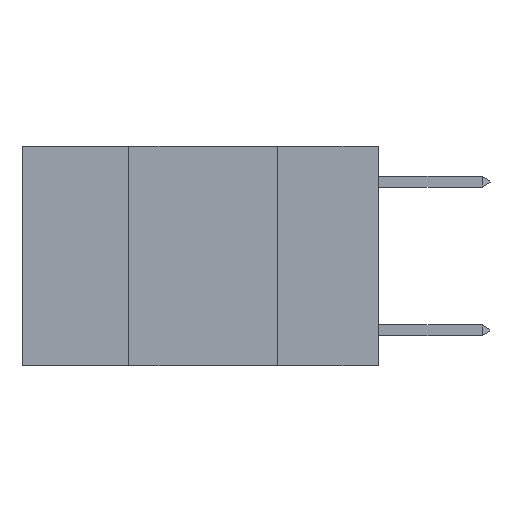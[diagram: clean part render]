
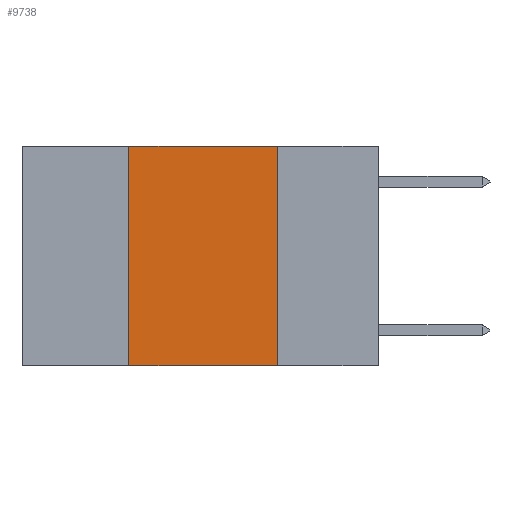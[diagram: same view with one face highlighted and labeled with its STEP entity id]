
A CAD part, left-side view. The second image highlights one B-rep face of the part: STEP entity #9738.
In plain terms, the highlighted planar face has unit normal (-1, 0, 0).
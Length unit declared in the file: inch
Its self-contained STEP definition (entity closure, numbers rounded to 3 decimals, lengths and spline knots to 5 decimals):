
#748 = VERTEX_POINT ( 'NONE', #5914 ) ;
#987 = CARTESIAN_POINT ( 'NONE',  ( 0., 0.17, -0.37 ) ) ;
#1013 = PLANE ( 'NONE',  #9119 ) ;
#1618 = DIRECTION ( 'NONE',  ( 0., 0., 1. ) ) ;
#1812 = DIRECTION ( 'NONE',  ( 1., 0., 0. ) ) ;
#1845 = CARTESIAN_POINT ( 'NONE',  ( 0., 0.6, -0.37 ) ) ;
#1848 = EDGE_CURVE ( 'NONE', #4637, #2134, #8633, .T. ) ;
#2129 = ORIENTED_EDGE ( 'NONE', *, *, #1848, .F. ) ;
#2134 = VERTEX_POINT ( 'NONE', #987 ) ;
#2303 = EDGE_CURVE ( 'NONE', #7152, #748, #2672, .T. ) ;
#2428 = VECTOR ( 'NONE', #5171, 39.37008 ) ;
#2672 = LINE ( 'NONE', #6162, #8623 ) ;
#2759 = ORIENTED_EDGE ( 'NONE', *, *, #5138, .F. ) ;
#2793 = EDGE_LOOP ( 'NONE', ( #2129, #2759, #3598, #3946 ) ) ;
#3598 = ORIENTED_EDGE ( 'NONE', *, *, #2303, .F. ) ;
#3946 = ORIENTED_EDGE ( 'NONE', *, *, #9270, .T. ) ;
#4184 = DIRECTION ( 'NONE',  ( 0., -1., 0. ) ) ;
#4637 = VERTEX_POINT ( 'NONE', #9753 ) ;
#5138 = EDGE_CURVE ( 'NONE', #748, #4637, #8863, .T. ) ;
#5171 = DIRECTION ( 'NONE',  ( 0., 0., -1. ) ) ;
#5399 = VECTOR ( 'NONE', #6515, 39.37008 ) ;
#5540 = CARTESIAN_POINT ( 'NONE',  ( 0., 0.42, -0.37 ) ) ;
#5815 = CARTESIAN_POINT ( 'NONE',  ( 0., 0.17, 0. ) ) ;
#5914 = CARTESIAN_POINT ( 'NONE',  ( 0., 0.42, 0. ) ) ;
#6162 = CARTESIAN_POINT ( 'NONE',  ( 0., 0.42, 0. ) ) ;
#6515 = DIRECTION ( 'NONE',  ( 0., -1., 0. ) ) ;
#6570 = VECTOR ( 'NONE', #4184, 39.37008 ) ;
#7152 = VERTEX_POINT ( 'NONE', #5540 ) ;
#7278 = DIRECTION ( 'NONE',  ( 0., 0., -1. ) ) ;
#8080 = CARTESIAN_POINT ( 'NONE',  ( 0., 0.6, 0. ) ) ;
#8623 = VECTOR ( 'NONE', #1618, 39.37008 ) ;
#8633 = LINE ( 'NONE', #5815, #2428 ) ;
#8790 = CARTESIAN_POINT ( 'NONE',  ( 0., 0.6, 0. ) ) ;
#8863 = LINE ( 'NONE', #8080, #6570 ) ;
#9119 = AXIS2_PLACEMENT_3D ( 'NONE', #8790, #1812, #7278 ) ;
#9270 = EDGE_CURVE ( 'NONE', #7152, #2134, #9526, .T. ) ;
#9515 = FACE_OUTER_BOUND ( 'NONE', #2793, .T. ) ;
#9526 = LINE ( 'NONE', #1845, #5399 ) ;
#9738 = ADVANCED_FACE ( 'NONE', ( #9515 ), #1013, .F. ) ;
#9753 = CARTESIAN_POINT ( 'NONE',  ( 0., 0.17, 0. ) ) ;
